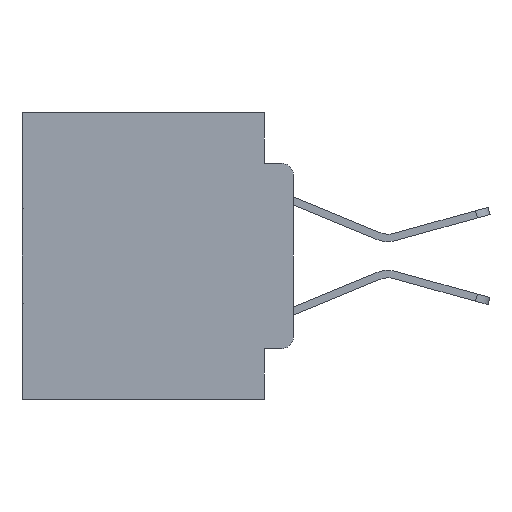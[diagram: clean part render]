
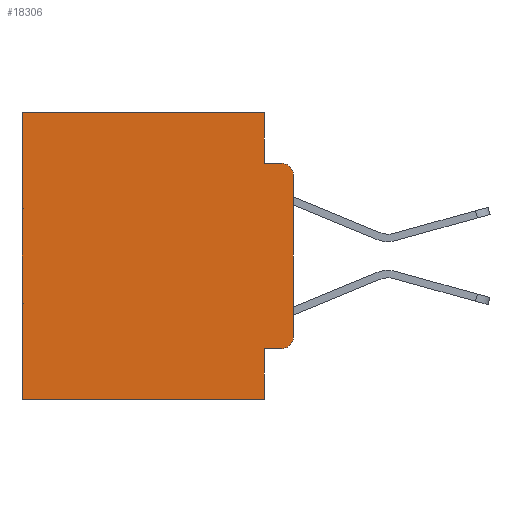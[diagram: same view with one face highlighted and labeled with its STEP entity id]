
A CAD part, left-side view. The second image highlights one B-rep face of the part: STEP entity #18306.
In plain terms, the highlighted planar face has unit normal (-1, 0, 0).
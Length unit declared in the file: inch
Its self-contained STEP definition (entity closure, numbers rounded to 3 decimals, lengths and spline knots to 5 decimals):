
#222 = DIRECTION ( 'NONE',  ( 0., 0., -1. ) ) ;
#1182 = CARTESIAN_POINT ( 'NONE',  ( 0.298, 0., -0.1085 ) ) ;
#1225 = VECTOR ( 'NONE', #6236, 39.37008 ) ;
#1235 = CARTESIAN_POINT ( 'NONE',  ( 0.298, 0.473, 0. ) ) ;
#1248 = VERTEX_POINT ( 'NONE', #1182 ) ;
#1428 = EDGE_CURVE ( 'NONE', #26849, #23534, #8702, .T. ) ;
#1658 = DIRECTION ( 'NONE',  ( 0., 0., -1. ) ) ;
#1804 = DIRECTION ( 'NONE',  ( 0., 0., -1. ) ) ;
#3068 = EDGE_CURVE ( 'NONE', #29526, #26849, #13677, .T. ) ;
#3171 = DIRECTION ( 'NONE',  ( 0., 0., -1. ) ) ;
#3178 = VECTOR ( 'NONE', #3171, 39.37008 ) ;
#3390 = EDGE_LOOP ( 'NONE', ( #14703, #26094, #5657, #4909, #28576, #27884, #21133, #8896, #18260, #29605 ) ) ;
#3719 = CARTESIAN_POINT ( 'NONE',  ( 0.298, 0.051, -0.0885 ) ) ;
#4227 = CARTESIAN_POINT ( 'NONE',  ( 0.298, 0.051, 0. ) ) ;
#4697 = VECTOR ( 'NONE', #18714, 39.37008 ) ;
#4814 = VERTEX_POINT ( 'NONE', #19383 ) ;
#4909 = ORIENTED_EDGE ( 'NONE', *, *, #12452, .F. ) ;
#5283 = VERTEX_POINT ( 'NONE', #16471 ) ;
#5437 = LINE ( 'NONE', #23214, #4697 ) ;
#5657 = ORIENTED_EDGE ( 'NONE', *, *, #18591, .F. ) ;
#6236 = DIRECTION ( 'NONE',  ( 0., -1., 0. ) ) ;
#6901 = VERTEX_POINT ( 'NONE', #16128 ) ;
#8212 = EDGE_CURVE ( 'NONE', #20367, #17771, #18907, .T. ) ;
#8269 = AXIS2_PLACEMENT_3D ( 'NONE', #29233, #15673, #1658 ) ;
#8283 = VECTOR ( 'NONE', #27500, 39.37008 ) ;
#8702 = CIRCLE ( 'NONE', #17339, 0.02 ) ;
#8896 = ORIENTED_EDGE ( 'NONE', *, *, #9330, .F. ) ;
#9168 = CARTESIAN_POINT ( 'NONE',  ( 0.298, 0., -0.5 ) ) ;
#9330 = EDGE_CURVE ( 'NONE', #29526, #6901, #13823, .T. ) ;
#9489 = CARTESIAN_POINT ( 'NONE',  ( 0.298, 0., -0.3915 ) ) ;
#9647 = LINE ( 'NONE', #23359, #15114 ) ;
#9752 = LINE ( 'NONE', #9168, #8283 ) ;
#10639 = CARTESIAN_POINT ( 'NONE',  ( 0.298, 0.051, -0.4115 ) ) ;
#10880 = EDGE_CURVE ( 'NONE', #17771, #4814, #26957, .T. ) ;
#10982 = DIRECTION ( 'NONE',  ( 0., 0., -1. ) ) ;
#11601 = DIRECTION ( 'NONE',  ( 0., 1., 0. ) ) ;
#12452 = EDGE_CURVE ( 'NONE', #20367, #13412, #9647, .T. ) ;
#12699 = FACE_OUTER_BOUND ( 'NONE', #3390, .T. ) ;
#12806 = VECTOR ( 'NONE', #11601, 39.37008 ) ;
#12900 = CARTESIAN_POINT ( 'NONE',  ( 0.298, 0.051, -0.4115 ) ) ;
#13136 = CARTESIAN_POINT ( 'NONE',  ( 0.298, 0.02, -0.3915 ) ) ;
#13412 = VERTEX_POINT ( 'NONE', #3719 ) ;
#13677 = LINE ( 'NONE', #10639, #1225 ) ;
#13823 = LINE ( 'NONE', #4227, #25266 ) ;
#14237 = CARTESIAN_POINT ( 'NONE',  ( 0.298, 0.051, 0. ) ) ;
#14614 = DIRECTION ( 'NONE',  ( 0., 0., -1. ) ) ;
#14703 = ORIENTED_EDGE ( 'NONE', *, *, #26234, .F. ) ;
#14996 = AXIS2_PLACEMENT_3D ( 'NONE', #24605, #24706, #10982 ) ;
#15114 = VECTOR ( 'NONE', #222, 39.37008 ) ;
#15673 = DIRECTION ( 'NONE',  ( -1., 0., 0. ) ) ;
#16128 = CARTESIAN_POINT ( 'NONE',  ( 0.298, 0.051, -0.5 ) ) ;
#16471 = CARTESIAN_POINT ( 'NONE',  ( 0.298, 0.02, -0.0885 ) ) ;
#16487 = CIRCLE ( 'NONE', #8269, 0.02 ) ;
#17068 = CARTESIAN_POINT ( 'NONE',  ( 0.298, 0.473, 0. ) ) ;
#17280 = CARTESIAN_POINT ( 'NONE',  ( 0.298, 0., 0. ) ) ;
#17339 = AXIS2_PLACEMENT_3D ( 'NONE', #13136, #26473, #14614 ) ;
#17628 = CARTESIAN_POINT ( 'NONE',  ( 0.298, 0.02, -0.4115 ) ) ;
#17771 = VERTEX_POINT ( 'NONE', #1235 ) ;
#18260 = ORIENTED_EDGE ( 'NONE', *, *, #3068, .T. ) ;
#18306 = ADVANCED_FACE ( 'NONE', ( #12699 ), #22422, .F. ) ;
#18591 = EDGE_CURVE ( 'NONE', #13412, #5283, #5437, .T. ) ;
#18714 = DIRECTION ( 'NONE',  ( 0., -1., 0. ) ) ;
#18907 = LINE ( 'NONE', #25307, #12806 ) ;
#19383 = CARTESIAN_POINT ( 'NONE',  ( 0.298, 0.473, -0.5 ) ) ;
#19558 = DIRECTION ( 'NONE',  ( 0., 0., -1. ) ) ;
#20103 = EDGE_CURVE ( 'NONE', #1248, #5283, #16487, .T. ) ;
#20367 = VERTEX_POINT ( 'NONE', #14237 ) ;
#20777 = VECTOR ( 'NONE', #19558, 39.37008 ) ;
#21133 = ORIENTED_EDGE ( 'NONE', *, *, #24624, .F. ) ;
#21509 = LINE ( 'NONE', #17280, #20777 ) ;
#22422 = PLANE ( 'NONE',  #14996 ) ;
#23214 = CARTESIAN_POINT ( 'NONE',  ( 0.298, 0.051, -0.0885 ) ) ;
#23359 = CARTESIAN_POINT ( 'NONE',  ( 0.298, 0.051, 0. ) ) ;
#23534 = VERTEX_POINT ( 'NONE', #9489 ) ;
#24605 = CARTESIAN_POINT ( 'NONE',  ( 0.298, 0., 0. ) ) ;
#24624 = EDGE_CURVE ( 'NONE', #6901, #4814, #9752, .T. ) ;
#24706 = DIRECTION ( 'NONE',  ( 1., 0., 0. ) ) ;
#25266 = VECTOR ( 'NONE', #1804, 39.37008 ) ;
#25307 = CARTESIAN_POINT ( 'NONE',  ( 0.298, 0., 0. ) ) ;
#26094 = ORIENTED_EDGE ( 'NONE', *, *, #20103, .T. ) ;
#26234 = EDGE_CURVE ( 'NONE', #1248, #23534, #21509, .T. ) ;
#26473 = DIRECTION ( 'NONE',  ( -1., 0., 0. ) ) ;
#26849 = VERTEX_POINT ( 'NONE', #17628 ) ;
#26957 = LINE ( 'NONE', #17068, #3178 ) ;
#27500 = DIRECTION ( 'NONE',  ( 0., 1., 0. ) ) ;
#27884 = ORIENTED_EDGE ( 'NONE', *, *, #10880, .T. ) ;
#28576 = ORIENTED_EDGE ( 'NONE', *, *, #8212, .T. ) ;
#29233 = CARTESIAN_POINT ( 'NONE',  ( 0.298, 0.02, -0.1085 ) ) ;
#29526 = VERTEX_POINT ( 'NONE', #12900 ) ;
#29605 = ORIENTED_EDGE ( 'NONE', *, *, #1428, .T. ) ;
